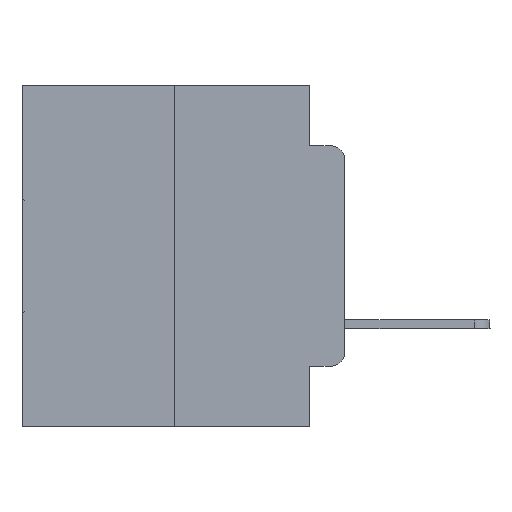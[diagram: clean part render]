
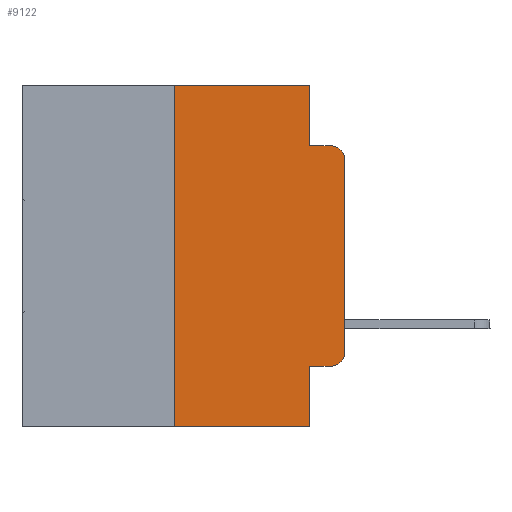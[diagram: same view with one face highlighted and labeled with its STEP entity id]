
A CAD part, left-side view. The second image highlights one B-rep face of the part: STEP entity #9122.
In plain terms, the highlighted planar face has unit normal (-1, 0, 0).
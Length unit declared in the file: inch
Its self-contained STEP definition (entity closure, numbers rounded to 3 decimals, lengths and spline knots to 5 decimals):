
#5 = LINE ( 'NONE', #26736, #19646 ) ;
#936 = DIRECTION ( 'NONE',  ( -1., 0., 0. ) ) ;
#1587 = CIRCLE ( 'NONE', #22651, 0.02 ) ;
#1739 = DIRECTION ( 'NONE',  ( 1., 0., 0. ) ) ;
#2203 = ORIENTED_EDGE ( 'NONE', *, *, #9887, .F. ) ;
#3023 = ORIENTED_EDGE ( 'NONE', *, *, #22650, .T. ) ;
#3657 = VERTEX_POINT ( 'NONE', #24787 ) ;
#3715 = LINE ( 'NONE', #22712, #4736 ) ;
#4469 = CIRCLE ( 'NONE', #11593, 0.02 ) ;
#4627 = ORIENTED_EDGE ( 'NONE', *, *, #15973, .T. ) ;
#4736 = VECTOR ( 'NONE', #22616, 39.37008 ) ;
#4879 = LINE ( 'NONE', #27592, #17869 ) ;
#5812 = VERTEX_POINT ( 'NONE', #25185 ) ;
#6495 = DIRECTION ( 'NONE',  ( 0., -1., 0. ) ) ;
#6590 = EDGE_CURVE ( 'NONE', #24543, #28506, #8848, .T. ) ;
#6726 = CARTESIAN_POINT ( 'NONE',  ( 0., 0.02, -0.4115 ) ) ;
#7436 = LINE ( 'NONE', #12063, #19024 ) ;
#7838 = DIRECTION ( 'NONE',  ( 0., 0., -1. ) ) ;
#8172 = EDGE_CURVE ( 'NONE', #3657, #17967, #3715, .T. ) ;
#8264 = EDGE_CURVE ( 'NONE', #15326, #3657, #1587, .T. ) ;
#8300 = CARTESIAN_POINT ( 'NONE',  ( 0., 0.051, -0.0885 ) ) ;
#8675 = CARTESIAN_POINT ( 'NONE',  ( 0., 0.25, 0. ) ) ;
#8686 = CARTESIAN_POINT ( 'NONE',  ( 0., 0.051, -0.0885 ) ) ;
#8848 = LINE ( 'NONE', #8675, #28097 ) ;
#8861 = DIRECTION ( 'NONE',  ( 0., -1., 0. ) ) ;
#9122 = ADVANCED_FACE ( 'NONE', ( #16951 ), #28604, .F. ) ;
#9826 = CARTESIAN_POINT ( 'NONE',  ( 0., 0.02, -0.1085 ) ) ;
#9887 = EDGE_CURVE ( 'NONE', #26840, #5812, #13428, .T. ) ;
#10033 = CARTESIAN_POINT ( 'NONE',  ( 0., 0.051, 0. ) ) ;
#10114 = CARTESIAN_POINT ( 'NONE',  ( 0., 0.051, -0.4115 ) ) ;
#10659 = VECTOR ( 'NONE', #6495, 39.37008 ) ;
#11184 = CARTESIAN_POINT ( 'NONE',  ( 0., 0.051, -0.4115 ) ) ;
#11305 = ORIENTED_EDGE ( 'NONE', *, *, #8172, .T. ) ;
#11593 = AXIS2_PLACEMENT_3D ( 'NONE', #9826, #936, #7838 ) ;
#12063 = CARTESIAN_POINT ( 'NONE',  ( 0., 0.473, 0. ) ) ;
#12820 = VERTEX_POINT ( 'NONE', #14352 ) ;
#13169 = ORIENTED_EDGE ( 'NONE', *, *, #19499, .T. ) ;
#13216 = DIRECTION ( 'NONE',  ( 0., 0., -1. ) ) ;
#13428 = LINE ( 'NONE', #8300, #10659 ) ;
#14352 = CARTESIAN_POINT ( 'NONE',  ( 0., 0.051, -0.5 ) ) ;
#14377 = LINE ( 'NONE', #18914, #29052 ) ;
#14615 = ORIENTED_EDGE ( 'NONE', *, *, #8264, .T. ) ;
#14739 = EDGE_CURVE ( 'NONE', #15998, #26840, #4879, .T. ) ;
#14977 = EDGE_CURVE ( 'NONE', #15299, #12820, #14377, .T. ) ;
#15228 = CARTESIAN_POINT ( 'NONE',  ( 0., 0.473, 0. ) ) ;
#15299 = VERTEX_POINT ( 'NONE', #11184 ) ;
#15326 = VERTEX_POINT ( 'NONE', #6726 ) ;
#15491 = CARTESIAN_POINT ( 'NONE',  ( 0., 0.02, -0.3915 ) ) ;
#15973 = EDGE_CURVE ( 'NONE', #17967, #5812, #4469, .T. ) ;
#15998 = VERTEX_POINT ( 'NONE', #10033 ) ;
#16713 = DIRECTION ( 'NONE',  ( 0., -1., 0. ) ) ;
#16951 = FACE_OUTER_BOUND ( 'NONE', #18708, .T. ) ;
#17406 = CARTESIAN_POINT ( 'NONE',  ( 0., 0.25, -0.5 ) ) ;
#17869 = VECTOR ( 'NONE', #25454, 39.37008 ) ;
#17967 = VERTEX_POINT ( 'NONE', #27435 ) ;
#18708 = EDGE_LOOP ( 'NONE', ( #11305, #4627, #2203, #24427, #19954, #26770, #3023, #23456, #13169, #14615 ) ) ;
#18914 = CARTESIAN_POINT ( 'NONE',  ( 0., 0.051, 0. ) ) ;
#19024 = VECTOR ( 'NONE', #23084, 39.37008 ) ;
#19499 = EDGE_CURVE ( 'NONE', #15299, #15326, #21064, .T. ) ;
#19646 = VECTOR ( 'NONE', #8861, 39.37008 ) ;
#19688 = DIRECTION ( 'NONE',  ( 0., 0., -1. ) ) ;
#19954 = ORIENTED_EDGE ( 'NONE', *, *, #27610, .F. ) ;
#21064 = LINE ( 'NONE', #10114, #21775 ) ;
#21273 = DIRECTION ( 'NONE',  ( 0., 0., -1. ) ) ;
#21775 = VECTOR ( 'NONE', #16713, 39.37008 ) ;
#21964 = DIRECTION ( 'NONE',  ( 0., 0., 1. ) ) ;
#22616 = DIRECTION ( 'NONE',  ( 0., 0., 1. ) ) ;
#22650 = EDGE_CURVE ( 'NONE', #24543, #12820, #5, .T. ) ;
#22651 = AXIS2_PLACEMENT_3D ( 'NONE', #15491, #29051, #13216 ) ;
#22712 = CARTESIAN_POINT ( 'NONE',  ( 0., 0., 0. ) ) ;
#23084 = DIRECTION ( 'NONE',  ( 0., -1., 0. ) ) ;
#23456 = ORIENTED_EDGE ( 'NONE', *, *, #14977, .F. ) ;
#24167 = AXIS2_PLACEMENT_3D ( 'NONE', #15228, #1739, #19688 ) ;
#24427 = ORIENTED_EDGE ( 'NONE', *, *, #14739, .F. ) ;
#24543 = VERTEX_POINT ( 'NONE', #17406 ) ;
#24787 = CARTESIAN_POINT ( 'NONE',  ( 0., 0., -0.3915 ) ) ;
#25185 = CARTESIAN_POINT ( 'NONE',  ( 0., 0.02, -0.0885 ) ) ;
#25454 = DIRECTION ( 'NONE',  ( 0., 0., -1. ) ) ;
#26383 = CARTESIAN_POINT ( 'NONE',  ( 0., 0.25, 0. ) ) ;
#26736 = CARTESIAN_POINT ( 'NONE',  ( 0., 0.473, -0.5 ) ) ;
#26770 = ORIENTED_EDGE ( 'NONE', *, *, #6590, .F. ) ;
#26840 = VERTEX_POINT ( 'NONE', #8686 ) ;
#27435 = CARTESIAN_POINT ( 'NONE',  ( 0., 0., -0.1085 ) ) ;
#27592 = CARTESIAN_POINT ( 'NONE',  ( 0., 0.051, 0. ) ) ;
#27610 = EDGE_CURVE ( 'NONE', #28506, #15998, #7436, .T. ) ;
#28097 = VECTOR ( 'NONE', #21964, 39.37008 ) ;
#28506 = VERTEX_POINT ( 'NONE', #26383 ) ;
#28604 = PLANE ( 'NONE',  #24167 ) ;
#29051 = DIRECTION ( 'NONE',  ( -1., 0., 0. ) ) ;
#29052 = VECTOR ( 'NONE', #21273, 39.37008 ) ;
